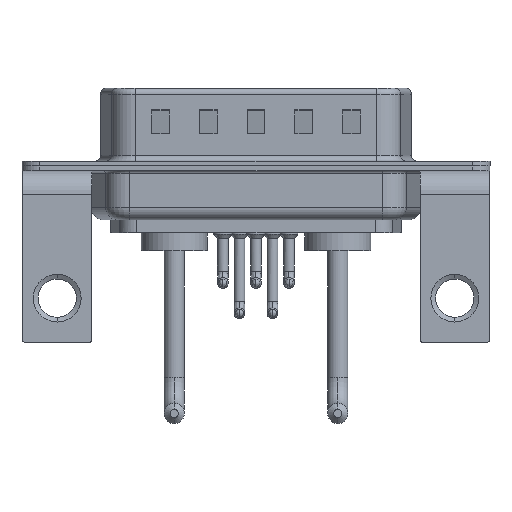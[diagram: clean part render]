
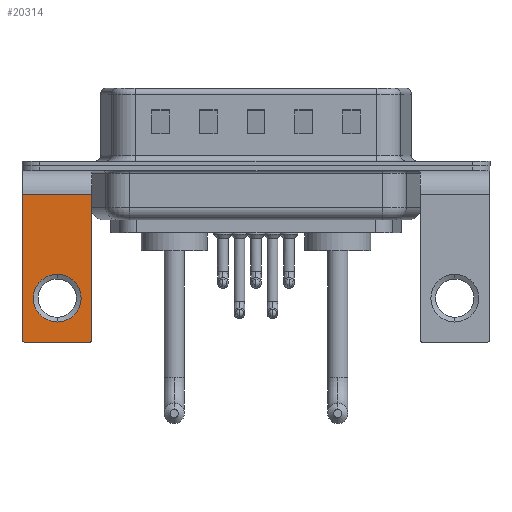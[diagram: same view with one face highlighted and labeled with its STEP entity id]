
A CAD part, front view. The second image highlights one B-rep face of the part: STEP entity #20314.
In plain terms, the highlighted planar face has unit normal (0, -1, 0).
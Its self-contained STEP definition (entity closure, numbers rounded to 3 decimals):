
#151 = CARTESIAN_POINT ( 'NONE',  ( 2.65, -6.25, -14.8 ) ) ;
#599 = VERTEX_POINT ( 'NONE', #6554 ) ;
#972 = DIRECTION ( 'NONE',  ( 0., 1., 0. ) ) ;
#1161 = PLANE ( 'NONE',  #12724 ) ;
#1226 = EDGE_CURVE ( 'NONE', #5095, #21274, #10369, .T. ) ;
#1621 = DIRECTION ( 'NONE',  ( 0., -1., 0. ) ) ;
#1698 = DIRECTION ( 'NONE',  ( -1., 0., 0. ) ) ;
#1916 = ORIENTED_EDGE ( 'NONE', *, *, #18637, .T. ) ;
#2484 = CIRCLE ( 'NONE', #13071, 0.25 ) ;
#3030 = DIRECTION ( 'NONE',  ( 0., 0., 1. ) ) ;
#3037 = VERTEX_POINT ( 'NONE', #17610 ) ;
#3076 = VECTOR ( 'NONE', #20989, 1000. ) ;
#3082 = ORIENTED_EDGE ( 'NONE', *, *, #4331, .T. ) ;
#3987 = DIRECTION ( 'NONE',  ( 0., 0., 1. ) ) ;
#4331 = EDGE_CURVE ( 'NONE', #15719, #9494, #5386, .T. ) ;
#4987 = VERTEX_POINT ( 'NONE', #151 ) ;
#5095 = VERTEX_POINT ( 'NONE', #7458 ) ;
#5386 = CIRCLE ( 'NONE', #14212, 2. ) ;
#5911 = EDGE_CURVE ( 'NONE', #9494, #15719, #11411, .T. ) ;
#6170 = DIRECTION ( 'NONE',  ( 0., 0., 1. ) ) ;
#6554 = CARTESIAN_POINT ( 'NONE',  ( -2.65, -6.25, -14.8 ) ) ;
#6814 = ORIENTED_EDGE ( 'NONE', *, *, #7972, .F. ) ;
#7023 = EDGE_LOOP ( 'NONE', ( #1916, #10118, #6814, #8886, #7772, #15725 ) ) ;
#7063 = LINE ( 'NONE', #13801, #3076 ) ;
#7458 = CARTESIAN_POINT ( 'NONE',  ( 2.9, -6.25, -2.4 ) ) ;
#7753 = CIRCLE ( 'NONE', #10920, 0.25 ) ;
#7772 = ORIENTED_EDGE ( 'NONE', *, *, #14183, .F. ) ;
#7927 = LINE ( 'NONE', #16641, #10977 ) ;
#7972 = EDGE_CURVE ( 'NONE', #4987, #599, #15119, .T. ) ;
#8886 = ORIENTED_EDGE ( 'NONE', *, *, #18595, .T. ) ;
#9190 = DIRECTION ( 'NONE',  ( 0., 0., 1. ) ) ;
#9273 = CARTESIAN_POINT ( 'NONE',  ( 2.9, -6.25, -2.4 ) ) ;
#9488 = ORIENTED_EDGE ( 'NONE', *, *, #5911, .T. ) ;
#9494 = VERTEX_POINT ( 'NONE', #18049 ) ;
#10027 = CARTESIAN_POINT ( 'NONE',  ( 2.9, -6.25, -2.4 ) ) ;
#10118 = ORIENTED_EDGE ( 'NONE', *, *, #10139, .T. ) ;
#10139 = EDGE_CURVE ( 'NONE', #18927, #599, #7753, .T. ) ;
#10295 = EDGE_LOOP ( 'NONE', ( #9488, #3082 ) ) ;
#10369 = LINE ( 'NONE', #10027, #14296 ) ;
#10920 = AXIS2_PLACEMENT_3D ( 'NONE', #18127, #1621, #11572 ) ;
#10977 = VECTOR ( 'NONE', #14761, 1000. ) ;
#11340 = CARTESIAN_POINT ( 'NONE',  ( 0., -6.25, -9.07 ) ) ;
#11411 = CIRCLE ( 'NONE', #12481, 2. ) ;
#11572 = DIRECTION ( 'NONE',  ( 0., 0., 1. ) ) ;
#12481 = AXIS2_PLACEMENT_3D ( 'NONE', #17354, #20888, #3987 ) ;
#12724 = AXIS2_PLACEMENT_3D ( 'NONE', #9273, #14765, #6170 ) ;
#13071 = AXIS2_PLACEMENT_3D ( 'NONE', #18084, #21403, #3030 ) ;
#13793 = VECTOR ( 'NONE', #20203, 1000. ) ;
#13801 = CARTESIAN_POINT ( 'NONE',  ( 2.9, -6.25, -2.4 ) ) ;
#14183 = EDGE_CURVE ( 'NONE', #5095, #3037, #7063, .T. ) ;
#14212 = AXIS2_PLACEMENT_3D ( 'NONE', #19243, #972, #9190 ) ;
#14296 = VECTOR ( 'NONE', #1698, 1000. ) ;
#14318 = CARTESIAN_POINT ( 'NONE',  ( -2.9, -6.25, -14.55 ) ) ;
#14586 = CARTESIAN_POINT ( 'NONE',  ( -2.9, -6.25, -2.4 ) ) ;
#14761 = DIRECTION ( 'NONE',  ( 0., 0., -1. ) ) ;
#14765 = DIRECTION ( 'NONE',  ( 0., 1., 0. ) ) ;
#15119 = LINE ( 'NONE', #21869, #13793 ) ;
#15719 = VERTEX_POINT ( 'NONE', #11340 ) ;
#15725 = ORIENTED_EDGE ( 'NONE', *, *, #1226, .T. ) ;
#16317 = FACE_OUTER_BOUND ( 'NONE', #7023, .T. ) ;
#16641 = CARTESIAN_POINT ( 'NONE',  ( -2.9, -6.25, -2.4 ) ) ;
#17330 = FACE_BOUND ( 'NONE', #10295, .T. ) ;
#17354 = CARTESIAN_POINT ( 'NONE',  ( 0., -6.25, -11.07 ) ) ;
#17610 = CARTESIAN_POINT ( 'NONE',  ( 2.9, -6.25, -14.55 ) ) ;
#18049 = CARTESIAN_POINT ( 'NONE',  ( 0., -6.25, -13.07 ) ) ;
#18084 = CARTESIAN_POINT ( 'NONE',  ( 2.65, -6.25, -14.55 ) ) ;
#18127 = CARTESIAN_POINT ( 'NONE',  ( -2.65, -6.25, -14.55 ) ) ;
#18595 = EDGE_CURVE ( 'NONE', #4987, #3037, #2484, .T. ) ;
#18637 = EDGE_CURVE ( 'NONE', #21274, #18927, #7927, .T. ) ;
#18927 = VERTEX_POINT ( 'NONE', #14318 ) ;
#19243 = CARTESIAN_POINT ( 'NONE',  ( 0., -6.25, -11.07 ) ) ;
#20203 = DIRECTION ( 'NONE',  ( -1., 0., 0. ) ) ;
#20314 = ADVANCED_FACE ( 'NONE', ( #17330, #16317 ), #1161, .F. ) ;
#20888 = DIRECTION ( 'NONE',  ( 0., 1., 0. ) ) ;
#20989 = DIRECTION ( 'NONE',  ( 0., 0., -1. ) ) ;
#21274 = VERTEX_POINT ( 'NONE', #14586 ) ;
#21403 = DIRECTION ( 'NONE',  ( 0., -1., 0. ) ) ;
#21869 = CARTESIAN_POINT ( 'NONE',  ( 2.9, -6.25, -14.8 ) ) ;
